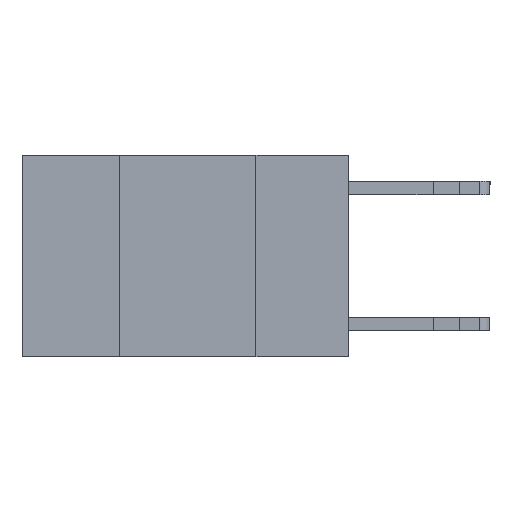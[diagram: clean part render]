
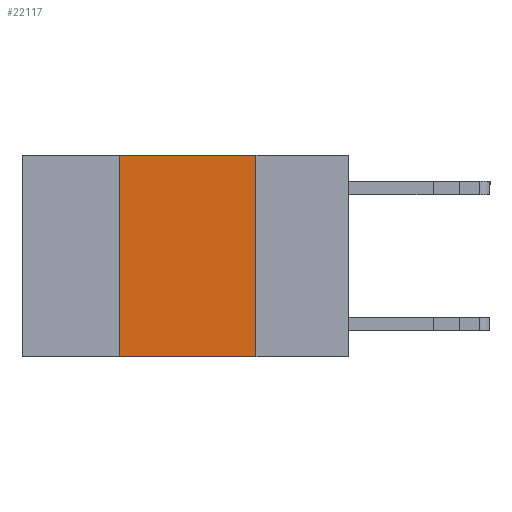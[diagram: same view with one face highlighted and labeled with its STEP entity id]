
A CAD part, left-side view. The second image highlights one B-rep face of the part: STEP entity #22117.
In plain terms, the highlighted planar face has unit normal (-1, 0, 0).
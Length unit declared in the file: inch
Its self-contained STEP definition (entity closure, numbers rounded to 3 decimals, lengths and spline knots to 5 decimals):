
#441 = CARTESIAN_POINT ( 'NONE',  ( 0., 0.17, 0. ) ) ;
#1547 = CARTESIAN_POINT ( 'NONE',  ( 0., 0.42, 0. ) ) ;
#1571 = CARTESIAN_POINT ( 'NONE',  ( 0., 0.42, 0. ) ) ;
#2288 = VECTOR ( 'NONE', #21873, 39.37008 ) ;
#3523 = PLANE ( 'NONE',  #8710 ) ;
#5334 = DIRECTION ( 'NONE',  ( 0., 0., -1. ) ) ;
#7146 = CARTESIAN_POINT ( 'NONE',  ( 0., 0.6, 0. ) ) ;
#7555 = FACE_OUTER_BOUND ( 'NONE', #27376, .T. ) ;
#7825 = LINE ( 'NONE', #1547, #25554 ) ;
#8055 = EDGE_CURVE ( 'NONE', #11196, #23379, #15730, .T. ) ;
#8147 = EDGE_CURVE ( 'NONE', #22759, #15639, #7825, .T. ) ;
#8710 = AXIS2_PLACEMENT_3D ( 'NONE', #7146, #13636, #22462 ) ;
#8857 = LINE ( 'NONE', #9127, #23368 ) ;
#9127 = CARTESIAN_POINT ( 'NONE',  ( 0., 0.6, -0.37 ) ) ;
#11196 = VERTEX_POINT ( 'NONE', #441 ) ;
#12820 = EDGE_CURVE ( 'NONE', #15639, #11196, #26480, .T. ) ;
#13538 = ORIENTED_EDGE ( 'NONE', *, *, #8147, .F. ) ;
#13636 = DIRECTION ( 'NONE',  ( 1., 0., 0. ) ) ;
#15012 = ORIENTED_EDGE ( 'NONE', *, *, #12820, .F. ) ;
#15639 = VERTEX_POINT ( 'NONE', #1571 ) ;
#15730 = LINE ( 'NONE', #24387, #19304 ) ;
#17552 = CARTESIAN_POINT ( 'NONE',  ( 0., 0.6, 0. ) ) ;
#19304 = VECTOR ( 'NONE', #5334, 39.37008 ) ;
#19631 = EDGE_CURVE ( 'NONE', #22759, #23379, #8857, .T. ) ;
#21873 = DIRECTION ( 'NONE',  ( 0., -1., 0. ) ) ;
#22117 = ADVANCED_FACE ( 'NONE', ( #7555 ), #3523, .F. ) ;
#22462 = DIRECTION ( 'NONE',  ( 0., 0., -1. ) ) ;
#22759 = VERTEX_POINT ( 'NONE', #23767 ) ;
#23368 = VECTOR ( 'NONE', #24020, 39.37008 ) ;
#23379 = VERTEX_POINT ( 'NONE', #24298 ) ;
#23767 = CARTESIAN_POINT ( 'NONE',  ( 0., 0.42, -0.37 ) ) ;
#24020 = DIRECTION ( 'NONE',  ( 0., -1., 0. ) ) ;
#24298 = CARTESIAN_POINT ( 'NONE',  ( 0., 0.17, -0.37 ) ) ;
#24387 = CARTESIAN_POINT ( 'NONE',  ( 0., 0.17, 0. ) ) ;
#24640 = ORIENTED_EDGE ( 'NONE', *, *, #19631, .T. ) ;
#25077 = ORIENTED_EDGE ( 'NONE', *, *, #8055, .F. ) ;
#25554 = VECTOR ( 'NONE', #26757, 39.37008 ) ;
#26480 = LINE ( 'NONE', #17552, #2288 ) ;
#26757 = DIRECTION ( 'NONE',  ( 0., 0., 1. ) ) ;
#27376 = EDGE_LOOP ( 'NONE', ( #25077, #15012, #13538, #24640 ) ) ;
